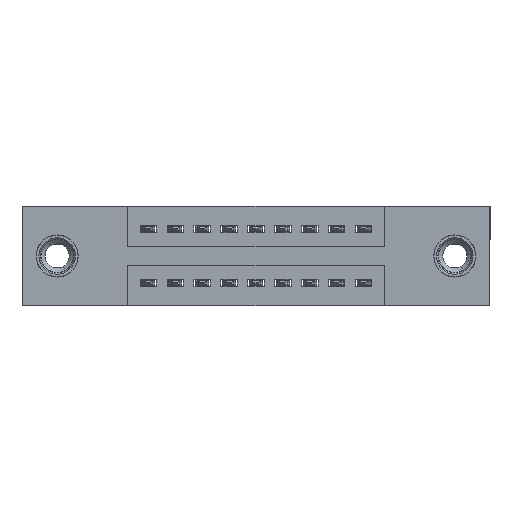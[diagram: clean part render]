
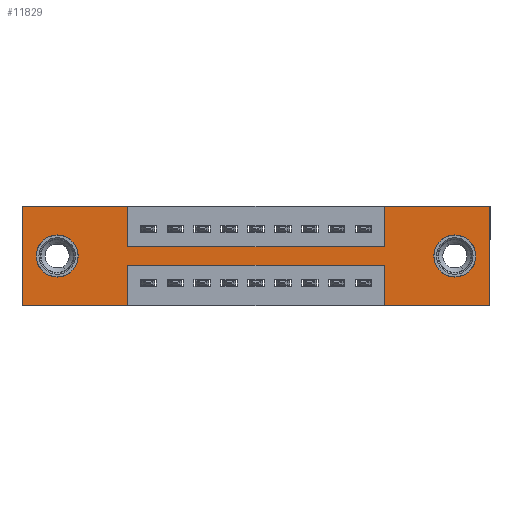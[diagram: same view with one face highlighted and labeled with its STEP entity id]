
A CAD part, front view. The second image highlights one B-rep face of the part: STEP entity #11829.
In plain terms, the highlighted planar face has unit normal (0, -1, 0).
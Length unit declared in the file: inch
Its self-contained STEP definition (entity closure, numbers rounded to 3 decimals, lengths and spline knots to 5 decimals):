
#107 = DIRECTION ( 'NONE',  ( 1., 0., 0. ) ) ;
#147 = CARTESIAN_POINT ( 'NONE',  ( 0., 0., 0. ) ) ;
#153 = VERTEX_POINT ( 'NONE', #2797 ) ;
#248 = EDGE_LOOP ( 'NONE', ( #2049, #1733 ) ) ;
#360 = CARTESIAN_POINT ( 'NONE',  ( 0.13, 0., -0.185 ) ) ;
#363 = VERTEX_POINT ( 'NONE', #8393 ) ;
#367 = CARTESIAN_POINT ( 'NONE',  ( 0.13, 0., -0.107 ) ) ;
#392 = PLANE ( 'NONE',  #3530 ) ;
#399 = LINE ( 'NONE', #14118, #12107 ) ;
#476 = VECTOR ( 'NONE', #5469, 39.37008 ) ;
#496 = CARTESIAN_POINT ( 'NONE',  ( 0.3925, 0., 0. ) ) ;
#651 = VECTOR ( 'NONE', #5830, 39.37008 ) ;
#711 = EDGE_CURVE ( 'NONE', #5109, #9778, #14377, .T. ) ;
#1320 = ORIENTED_EDGE ( 'NONE', *, *, #9723, .F. ) ;
#1547 = VECTOR ( 'NONE', #9591, 39.37008 ) ;
#1639 = ORIENTED_EDGE ( 'NONE', *, *, #7614, .F. ) ;
#1733 = ORIENTED_EDGE ( 'NONE', *, *, #5587, .T. ) ;
#1897 = ORIENTED_EDGE ( 'NONE', *, *, #13645, .F. ) ;
#2049 = ORIENTED_EDGE ( 'NONE', *, *, #8484, .T. ) ;
#2079 = LINE ( 'NONE', #13045, #14153 ) ;
#2369 = VECTOR ( 'NONE', #2696, 39.37008 ) ;
#2432 = CARTESIAN_POINT ( 'NONE',  ( 0., 0., -0.37 ) ) ;
#2474 = DIRECTION ( 'NONE',  ( 1., 0., 0. ) ) ;
#2551 = CARTESIAN_POINT ( 'NONE',  ( 0.3925, 0., -0.22 ) ) ;
#2592 = DIRECTION ( 'NONE',  ( -1., 0., 0. ) ) ;
#2672 = DIRECTION ( 'NONE',  ( 0., 0., -1. ) ) ;
#2696 = DIRECTION ( 'NONE',  ( 0., 0., 1. ) ) ;
#2702 = CARTESIAN_POINT ( 'NONE',  ( 1.605, 0., -0.185 ) ) ;
#2797 = CARTESIAN_POINT ( 'NONE',  ( 0.3925, 0., -0.15 ) ) ;
#3125 = LINE ( 'NONE', #14554, #1547 ) ;
#3170 = CIRCLE ( 'NONE', #8674, 0.078 ) ;
#3238 = CARTESIAN_POINT ( 'NONE',  ( 1.3425, 0., 0. ) ) ;
#3340 = CIRCLE ( 'NONE', #9116, 0.078 ) ;
#3366 = EDGE_CURVE ( 'NONE', #8190, #10433, #12342, .T. ) ;
#3431 = VERTEX_POINT ( 'NONE', #4945 ) ;
#3481 = ORIENTED_EDGE ( 'NONE', *, *, #13977, .F. ) ;
#3524 = VECTOR ( 'NONE', #107, 39.37008 ) ;
#3530 = AXIS2_PLACEMENT_3D ( 'NONE', #11799, #5504, #14371 ) ;
#3784 = CARTESIAN_POINT ( 'NONE',  ( 1.605, 0., -0.263 ) ) ;
#3864 = ORIENTED_EDGE ( 'NONE', *, *, #711, .F. ) ;
#3877 = DIRECTION ( 'NONE',  ( 0., 0., 1. ) ) ;
#3882 = VERTEX_POINT ( 'NONE', #11812 ) ;
#3967 = ORIENTED_EDGE ( 'NONE', *, *, #16057, .F. ) ;
#4061 = DIRECTION ( 'NONE',  ( 0., 0., -1. ) ) ;
#4167 = DIRECTION ( 'NONE',  ( 0., 1., 0. ) ) ;
#4234 = CARTESIAN_POINT ( 'NONE',  ( 0., 0., 0. ) ) ;
#4383 = ORIENTED_EDGE ( 'NONE', *, *, #4534, .F. ) ;
#4534 = EDGE_CURVE ( 'NONE', #4661, #153, #399, .T. ) ;
#4543 = CARTESIAN_POINT ( 'NONE',  ( 1.3425, 0., 0. ) ) ;
#4661 = VERTEX_POINT ( 'NONE', #496 ) ;
#4692 = FACE_OUTER_BOUND ( 'NONE', #8485, .T. ) ;
#4760 = ORIENTED_EDGE ( 'NONE', *, *, #10173, .T. ) ;
#4945 = CARTESIAN_POINT ( 'NONE',  ( 0., 0., -0.37 ) ) ;
#4969 = VECTOR ( 'NONE', #8293, 39.37008 ) ;
#4979 = CARTESIAN_POINT ( 'NONE',  ( 0., 0., 0. ) ) ;
#5109 = VERTEX_POINT ( 'NONE', #9940 ) ;
#5290 = CARTESIAN_POINT ( 'NONE',  ( 0.3925, 0., -0.37 ) ) ;
#5442 = ORIENTED_EDGE ( 'NONE', *, *, #8077, .T. ) ;
#5469 = DIRECTION ( 'NONE',  ( -1., 0., 0. ) ) ;
#5471 = ORIENTED_EDGE ( 'NONE', *, *, #12270, .F. ) ;
#5504 = DIRECTION ( 'NONE',  ( 0., -1., 0. ) ) ;
#5524 = VERTEX_POINT ( 'NONE', #147 ) ;
#5587 = EDGE_CURVE ( 'NONE', #11655, #15805, #3170, .T. ) ;
#5720 = EDGE_LOOP ( 'NONE', ( #5442, #4760 ) ) ;
#5830 = DIRECTION ( 'NONE',  ( 0., 0., 1. ) ) ;
#6095 = VERTEX_POINT ( 'NONE', #14419 ) ;
#6131 = LINE ( 'NONE', #14149, #2369 ) ;
#6142 = VERTEX_POINT ( 'NONE', #367 ) ;
#6319 = DIRECTION ( 'NONE',  ( 0., 1., 0. ) ) ;
#6757 = DIRECTION ( 'NONE',  ( 0., 0., 1. ) ) ;
#6809 = DIRECTION ( 'NONE',  ( 0., 1., 0. ) ) ;
#6912 = VECTOR ( 'NONE', #2672, 39.37008 ) ;
#7380 = VERTEX_POINT ( 'NONE', #12032 ) ;
#7559 = CARTESIAN_POINT ( 'NONE',  ( 1.605, 0., -0.107 ) ) ;
#7614 = EDGE_CURVE ( 'NONE', #10433, #7380, #13799, .T. ) ;
#7838 = CIRCLE ( 'NONE', #11631, 0.078 ) ;
#7845 = CARTESIAN_POINT ( 'NONE',  ( 0., 0., -0.37 ) ) ;
#8077 = EDGE_CURVE ( 'NONE', #6142, #6095, #15391, .T. ) ;
#8190 = VERTEX_POINT ( 'NONE', #14523 ) ;
#8293 = DIRECTION ( 'NONE',  ( 0., 0., 1. ) ) ;
#8340 = ORIENTED_EDGE ( 'NONE', *, *, #10147, .F. ) ;
#8393 = CARTESIAN_POINT ( 'NONE',  ( 0.3925, 0., -0.37 ) ) ;
#8434 = ORIENTED_EDGE ( 'NONE', *, *, #10372, .F. ) ;
#8455 = FACE_BOUND ( 'NONE', #5720, .T. ) ;
#8484 = EDGE_CURVE ( 'NONE', #15805, #11655, #7838, .T. ) ;
#8485 = EDGE_LOOP ( 'NONE', ( #12578, #1320, #8340, #3864, #1897, #1639, #15798, #8434, #4383, #5471, #3967, #3481 ) ) ;
#8674 = AXIS2_PLACEMENT_3D ( 'NONE', #2702, #6319, #11540 ) ;
#8724 = VECTOR ( 'NONE', #12597, 39.37008 ) ;
#9116 = AXIS2_PLACEMENT_3D ( 'NONE', #360, #6809, #6757 ) ;
#9284 = LINE ( 'NONE', #10058, #8724 ) ;
#9285 = CARTESIAN_POINT ( 'NONE',  ( 0., 0., 0. ) ) ;
#9591 = DIRECTION ( 'NONE',  ( 1., 0., 0. ) ) ;
#9723 = EDGE_CURVE ( 'NONE', #3882, #15760, #9284, .T. ) ;
#9778 = VERTEX_POINT ( 'NONE', #13147 ) ;
#9940 = CARTESIAN_POINT ( 'NONE',  ( 1.735, 0., -0.37 ) ) ;
#10058 = CARTESIAN_POINT ( 'NONE',  ( 0.3925, 0., -0.22 ) ) ;
#10147 = EDGE_CURVE ( 'NONE', #9778, #3882, #6131, .T. ) ;
#10173 = EDGE_CURVE ( 'NONE', #6095, #6142, #3340, .T. ) ;
#10356 = DIRECTION ( 'NONE',  ( 0., 0., -1. ) ) ;
#10372 = EDGE_CURVE ( 'NONE', #153, #8190, #3125, .T. ) ;
#10407 = CARTESIAN_POINT ( 'NONE',  ( 0.13, 0., -0.185 ) ) ;
#10433 = VERTEX_POINT ( 'NONE', #3238 ) ;
#11351 = VECTOR ( 'NONE', #2592, 39.37008 ) ;
#11540 = DIRECTION ( 'NONE',  ( 0., 0., -1. ) ) ;
#11631 = AXIS2_PLACEMENT_3D ( 'NONE', #11670, #4167, #10356 ) ;
#11651 = EDGE_CURVE ( 'NONE', #15760, #363, #16185, .T. ) ;
#11655 = VERTEX_POINT ( 'NONE', #3784 ) ;
#11670 = CARTESIAN_POINT ( 'NONE',  ( 1.605, 0., -0.185 ) ) ;
#11799 = CARTESIAN_POINT ( 'NONE',  ( 0., 0., -0.37 ) ) ;
#11812 = CARTESIAN_POINT ( 'NONE',  ( 1.3425, 0., -0.22 ) ) ;
#11829 = ADVANCED_FACE ( 'NONE', ( #12994, #8455, #4692 ), #392, .T. ) ;
#12032 = CARTESIAN_POINT ( 'NONE',  ( 1.735, 0., 0. ) ) ;
#12107 = VECTOR ( 'NONE', #4061, 39.37008 ) ;
#12178 = AXIS2_PLACEMENT_3D ( 'NONE', #10407, #12669, #3877 ) ;
#12270 = EDGE_CURVE ( 'NONE', #5524, #4661, #15959, .T. ) ;
#12342 = LINE ( 'NONE', #4543, #651 ) ;
#12578 = ORIENTED_EDGE ( 'NONE', *, *, #11651, .F. ) ;
#12597 = DIRECTION ( 'NONE',  ( -1., 0., 0. ) ) ;
#12669 = DIRECTION ( 'NONE',  ( 0., 1., 0. ) ) ;
#12938 = DIRECTION ( 'NONE',  ( 0., 0., -1. ) ) ;
#12994 = FACE_BOUND ( 'NONE', #248, .T. ) ;
#13045 = CARTESIAN_POINT ( 'NONE',  ( 1.735, 0., 0. ) ) ;
#13062 = LINE ( 'NONE', #9285, #4969 ) ;
#13147 = CARTESIAN_POINT ( 'NONE',  ( 1.3425, 0., -0.37 ) ) ;
#13335 = LINE ( 'NONE', #2432, #11351 ) ;
#13645 = EDGE_CURVE ( 'NONE', #7380, #5109, #2079, .T. ) ;
#13799 = LINE ( 'NONE', #4234, #3524 ) ;
#13977 = EDGE_CURVE ( 'NONE', #363, #3431, #13335, .T. ) ;
#14118 = CARTESIAN_POINT ( 'NONE',  ( 0.3925, 0., 0. ) ) ;
#14149 = CARTESIAN_POINT ( 'NONE',  ( 1.3425, 0., -0.37 ) ) ;
#14153 = VECTOR ( 'NONE', #12938, 39.37008 ) ;
#14371 = DIRECTION ( 'NONE',  ( 0., 0., -1. ) ) ;
#14377 = LINE ( 'NONE', #7845, #476 ) ;
#14419 = CARTESIAN_POINT ( 'NONE',  ( 0.13, 0., -0.263 ) ) ;
#14523 = CARTESIAN_POINT ( 'NONE',  ( 1.3425, 0., -0.15 ) ) ;
#14554 = CARTESIAN_POINT ( 'NONE',  ( 0.3925, 0., -0.15 ) ) ;
#15391 = CIRCLE ( 'NONE', #12178, 0.078 ) ;
#15760 = VERTEX_POINT ( 'NONE', #2551 ) ;
#15776 = VECTOR ( 'NONE', #2474, 39.37008 ) ;
#15798 = ORIENTED_EDGE ( 'NONE', *, *, #3366, .F. ) ;
#15805 = VERTEX_POINT ( 'NONE', #7559 ) ;
#15959 = LINE ( 'NONE', #4979, #15776 ) ;
#16057 = EDGE_CURVE ( 'NONE', #3431, #5524, #13062, .T. ) ;
#16185 = LINE ( 'NONE', #5290, #6912 ) ;
